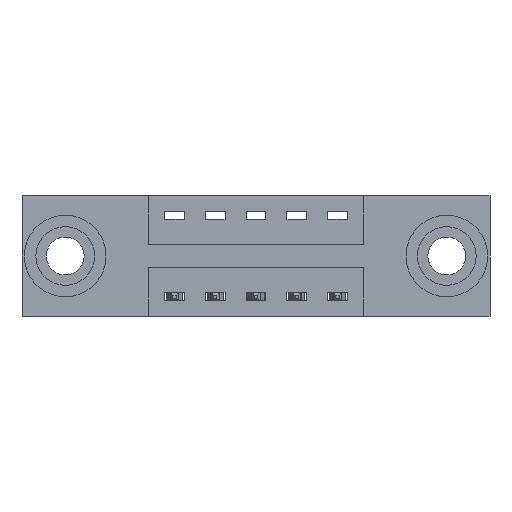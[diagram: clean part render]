
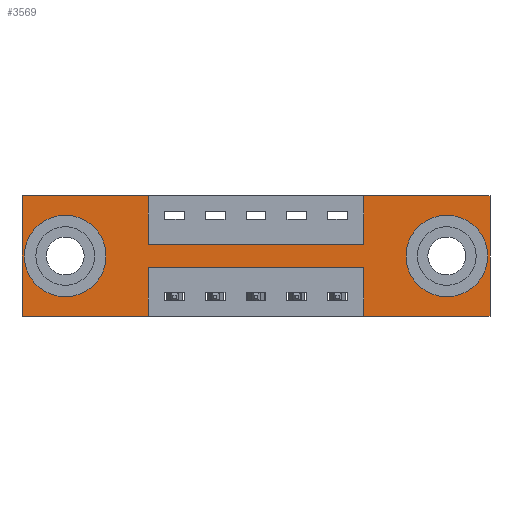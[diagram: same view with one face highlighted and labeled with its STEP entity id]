
A CAD part, front view. The second image highlights one B-rep face of the part: STEP entity #3569.
In plain terms, the highlighted planar face has unit normal (0, -1, 0).
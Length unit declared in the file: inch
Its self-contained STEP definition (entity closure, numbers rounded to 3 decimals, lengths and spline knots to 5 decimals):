
#14 = DIRECTION ( 'NONE',  ( 0., 1., 0. ) ) ;
#58 = VECTOR ( 'NONE', #2549, 39.37008 ) ;
#87 = DIRECTION ( 'NONE',  ( 0., 1., 0. ) ) ;
#312 = VERTEX_POINT ( 'NONE', #4707 ) ;
#434 = DIRECTION ( 'NONE',  ( 1., 0., 0. ) ) ;
#550 = DIRECTION ( 'NONE',  ( 0., 0., -1. ) ) ;
#617 = CARTESIAN_POINT ( 'NONE',  ( 0., 0., -0.37 ) ) ;
#631 = CIRCLE ( 'NONE', #5058, 0.078 ) ;
#636 = VECTOR ( 'NONE', #8516, 39.37008 ) ;
#1135 = VERTEX_POINT ( 'NONE', #1480 ) ;
#1148 = VERTEX_POINT ( 'NONE', #3266 ) ;
#1238 = VERTEX_POINT ( 'NONE', #4792 ) ;
#1344 = VECTOR ( 'NONE', #3670, 39.37008 ) ;
#1382 = CARTESIAN_POINT ( 'NONE',  ( 0., 0., -0.37 ) ) ;
#1480 = CARTESIAN_POINT ( 'NONE',  ( 1.0475, 0., 0. ) ) ;
#1633 = CIRCLE ( 'NONE', #2743, 0.078 ) ;
#1682 = LINE ( 'NONE', #617, #3852 ) ;
#1690 = EDGE_CURVE ( 'NONE', #5022, #4875, #1633, .T. ) ;
#1745 = VECTOR ( 'NONE', #2656, 39.37008 ) ;
#1761 = EDGE_CURVE ( 'NONE', #1135, #3083, #7922, .T. ) ;
#1864 = CARTESIAN_POINT ( 'NONE',  ( 0.3875, 0., -0.37 ) ) ;
#1916 = EDGE_LOOP ( 'NONE', ( #6002, #4593, #3584, #3527, #2947, #2757, #2307, #5243, #5201, #5235, #5082, #5350 ) ) ;
#1921 = CARTESIAN_POINT ( 'NONE',  ( 1.0475, 0., -0.37 ) ) ;
#1949 = CARTESIAN_POINT ( 'NONE',  ( 0., 0., -0.37 ) ) ;
#2166 = VECTOR ( 'NONE', #3898, 39.37008 ) ;
#2168 = CARTESIAN_POINT ( 'NONE',  ( 1.435, 0., 0. ) ) ;
#2193 = CARTESIAN_POINT ( 'NONE',  ( 0.3875, 0., -0.15 ) ) ;
#2196 = PLANE ( 'NONE',  #7880 ) ;
#2232 = CIRCLE ( 'NONE', #8319, 0.078 ) ;
#2291 = LINE ( 'NONE', #4595, #8593 ) ;
#2293 = EDGE_CURVE ( 'NONE', #8522, #1135, #6394, .T. ) ;
#2307 = ORIENTED_EDGE ( 'NONE', *, *, #2293, .F. ) ;
#2315 = FACE_BOUND ( 'NONE', #4770, .T. ) ;
#2337 = LINE ( 'NONE', #2193, #8637 ) ;
#2549 = DIRECTION ( 'NONE',  ( 0., 0., -1. ) ) ;
#2567 = LINE ( 'NONE', #3282, #58 ) ;
#2619 = CARTESIAN_POINT ( 'NONE',  ( 0.3875, 0., -0.22 ) ) ;
#2639 = CARTESIAN_POINT ( 'NONE',  ( 0.1325, 0., -0.263 ) ) ;
#2656 = DIRECTION ( 'NONE',  ( 0., 0., 1. ) ) ;
#2743 = AXIS2_PLACEMENT_3D ( 'NONE', #6141, #3408, #3191 ) ;
#2757 = ORIENTED_EDGE ( 'NONE', *, *, #1761, .F. ) ;
#2947 = ORIENTED_EDGE ( 'NONE', *, *, #8371, .F. ) ;
#3083 = VERTEX_POINT ( 'NONE', #2168 ) ;
#3154 = CARTESIAN_POINT ( 'NONE',  ( 0.3875, 0., 0. ) ) ;
#3191 = DIRECTION ( 'NONE',  ( 0., 0., 1. ) ) ;
#3193 = DIRECTION ( 'NONE',  ( 0., 0., -1. ) ) ;
#3266 = CARTESIAN_POINT ( 'NONE',  ( 1.3025, 0., -0.107 ) ) ;
#3282 = CARTESIAN_POINT ( 'NONE',  ( 0.3875, 0., -0.37 ) ) ;
#3408 = DIRECTION ( 'NONE',  ( 0., 1., 0. ) ) ;
#3461 = CARTESIAN_POINT ( 'NONE',  ( 1.0475, 0., 0. ) ) ;
#3478 = CARTESIAN_POINT ( 'NONE',  ( 0., 0., 0. ) ) ;
#3527 = ORIENTED_EDGE ( 'NONE', *, *, #4435, .F. ) ;
#3569 = ADVANCED_FACE ( 'NONE', ( #2315, #7407, #3978 ), #2196, .T. ) ;
#3582 = CARTESIAN_POINT ( 'NONE',  ( 0.3875, 0., -0.22 ) ) ;
#3584 = ORIENTED_EDGE ( 'NONE', *, *, #8078, .F. ) ;
#3670 = DIRECTION ( 'NONE',  ( 0., 0., -1. ) ) ;
#3748 = CIRCLE ( 'NONE', #7837, 0.078 ) ;
#3852 = VECTOR ( 'NONE', #5043, 39.37008 ) ;
#3898 = DIRECTION ( 'NONE',  ( 0., 0., 1. ) ) ;
#3944 = LINE ( 'NONE', #4159, #7181 ) ;
#3958 = EDGE_CURVE ( 'NONE', #7467, #1148, #3748, .T. ) ;
#3978 = FACE_OUTER_BOUND ( 'NONE', #1916, .T. ) ;
#4049 = DIRECTION ( 'NONE',  ( -1., 0., 0. ) ) ;
#4092 = ORIENTED_EDGE ( 'NONE', *, *, #3958, .T. ) ;
#4159 = CARTESIAN_POINT ( 'NONE',  ( 0., 0., 0. ) ) ;
#4255 = EDGE_LOOP ( 'NONE', ( #5183, #4677 ) ) ;
#4404 = LINE ( 'NONE', #1949, #7567 ) ;
#4421 = ORIENTED_EDGE ( 'NONE', *, *, #6792, .T. ) ;
#4435 = EDGE_CURVE ( 'NONE', #4826, #312, #1682, .T. ) ;
#4475 = CARTESIAN_POINT ( 'NONE',  ( 1.3025, 0., -0.185 ) ) ;
#4543 = CARTESIAN_POINT ( 'NONE',  ( 0.1325, 0., -0.185 ) ) ;
#4593 = ORIENTED_EDGE ( 'NONE', *, *, #8765, .F. ) ;
#4595 = CARTESIAN_POINT ( 'NONE',  ( 0.3875, 0., 0. ) ) ;
#4640 = EDGE_CURVE ( 'NONE', #5404, #5524, #2291, .T. ) ;
#4677 = ORIENTED_EDGE ( 'NONE', *, *, #8504, .T. ) ;
#4707 = CARTESIAN_POINT ( 'NONE',  ( 1.0475, 0., -0.37 ) ) ;
#4770 = EDGE_LOOP ( 'NONE', ( #4421, #4092 ) ) ;
#4792 = CARTESIAN_POINT ( 'NONE',  ( 1.0475, 0., -0.22 ) ) ;
#4826 = VERTEX_POINT ( 'NONE', #7833 ) ;
#4875 = VERTEX_POINT ( 'NONE', #2639 ) ;
#4951 = DIRECTION ( 'NONE',  ( 0., 1., 0. ) ) ;
#4991 = DIRECTION ( 'NONE',  ( 1., 0., 0. ) ) ;
#5022 = VERTEX_POINT ( 'NONE', #6173 ) ;
#5033 = CARTESIAN_POINT ( 'NONE',  ( 1.3025, 0., -0.263 ) ) ;
#5043 = DIRECTION ( 'NONE',  ( -1., 0., 0. ) ) ;
#5058 = AXIS2_PLACEMENT_3D ( 'NONE', #4475, #14, #5138 ) ;
#5082 = ORIENTED_EDGE ( 'NONE', *, *, #6207, .F. ) ;
#5138 = DIRECTION ( 'NONE',  ( 0., 0., -1. ) ) ;
#5183 = ORIENTED_EDGE ( 'NONE', *, *, #1690, .T. ) ;
#5195 = DIRECTION ( 'NONE',  ( 0., 0., 1. ) ) ;
#5201 = ORIENTED_EDGE ( 'NONE', *, *, #4640, .F. ) ;
#5235 = ORIENTED_EDGE ( 'NONE', *, *, #5640, .F. ) ;
#5243 = ORIENTED_EDGE ( 'NONE', *, *, #8278, .F. ) ;
#5279 = CARTESIAN_POINT ( 'NONE',  ( 0., 0., 0. ) ) ;
#5350 = ORIENTED_EDGE ( 'NONE', *, *, #5616, .F. ) ;
#5404 = VERTEX_POINT ( 'NONE', #3154 ) ;
#5524 = VERTEX_POINT ( 'NONE', #7776 ) ;
#5616 = EDGE_CURVE ( 'NONE', #7134, #7195, #4404, .T. ) ;
#5640 = EDGE_CURVE ( 'NONE', #7286, #5404, #3944, .T. ) ;
#6002 = ORIENTED_EDGE ( 'NONE', *, *, #7062, .F. ) ;
#6141 = CARTESIAN_POINT ( 'NONE',  ( 0.1325, 0., -0.185 ) ) ;
#6173 = CARTESIAN_POINT ( 'NONE',  ( 0.1325, 0., -0.107 ) ) ;
#6207 = EDGE_CURVE ( 'NONE', #7195, #7286, #7562, .T. ) ;
#6394 = LINE ( 'NONE', #3461, #7629 ) ;
#6466 = CARTESIAN_POINT ( 'NONE',  ( 1.0475, 0., -0.15 ) ) ;
#6673 = LINE ( 'NONE', #6941, #1344 ) ;
#6784 = DIRECTION ( 'NONE',  ( 0., 0., 1. ) ) ;
#6792 = EDGE_CURVE ( 'NONE', #1148, #7467, #631, .T. ) ;
#6893 = DIRECTION ( 'NONE',  ( 0., 0., -1. ) ) ;
#6941 = CARTESIAN_POINT ( 'NONE',  ( 1.435, 0., 0. ) ) ;
#7062 = EDGE_CURVE ( 'NONE', #8293, #7134, #2567, .T. ) ;
#7134 = VERTEX_POINT ( 'NONE', #1864 ) ;
#7148 = LINE ( 'NONE', #1921, #1745 ) ;
#7181 = VECTOR ( 'NONE', #434, 39.37008 ) ;
#7195 = VERTEX_POINT ( 'NONE', #7920 ) ;
#7229 = LINE ( 'NONE', #2619, #8628 ) ;
#7286 = VERTEX_POINT ( 'NONE', #3478 ) ;
#7322 = DIRECTION ( 'NONE',  ( -1., 0., 0. ) ) ;
#7407 = FACE_BOUND ( 'NONE', #4255, .T. ) ;
#7467 = VERTEX_POINT ( 'NONE', #5033 ) ;
#7562 = LINE ( 'NONE', #5279, #2166 ) ;
#7567 = VECTOR ( 'NONE', #7322, 39.37008 ) ;
#7629 = VECTOR ( 'NONE', #6784, 39.37008 ) ;
#7776 = CARTESIAN_POINT ( 'NONE',  ( 0.3875, 0., -0.15 ) ) ;
#7833 = CARTESIAN_POINT ( 'NONE',  ( 1.435, 0., -0.37 ) ) ;
#7837 = AXIS2_PLACEMENT_3D ( 'NONE', #8638, #4951, #550 ) ;
#7880 = AXIS2_PLACEMENT_3D ( 'NONE', #1382, #8674, #6893 ) ;
#7920 = CARTESIAN_POINT ( 'NONE',  ( 0., 0., -0.37 ) ) ;
#7922 = LINE ( 'NONE', #8497, #636 ) ;
#8078 = EDGE_CURVE ( 'NONE', #312, #1238, #7148, .T. ) ;
#8278 = EDGE_CURVE ( 'NONE', #5524, #8522, #2337, .T. ) ;
#8293 = VERTEX_POINT ( 'NONE', #3582 ) ;
#8319 = AXIS2_PLACEMENT_3D ( 'NONE', #4543, #87, #5195 ) ;
#8371 = EDGE_CURVE ( 'NONE', #3083, #4826, #6673, .T. ) ;
#8497 = CARTESIAN_POINT ( 'NONE',  ( 0., 0., 0. ) ) ;
#8504 = EDGE_CURVE ( 'NONE', #4875, #5022, #2232, .T. ) ;
#8516 = DIRECTION ( 'NONE',  ( 1., 0., 0. ) ) ;
#8522 = VERTEX_POINT ( 'NONE', #6466 ) ;
#8593 = VECTOR ( 'NONE', #3193, 39.37008 ) ;
#8628 = VECTOR ( 'NONE', #4049, 39.37008 ) ;
#8637 = VECTOR ( 'NONE', #4991, 39.37008 ) ;
#8638 = CARTESIAN_POINT ( 'NONE',  ( 1.3025, 0., -0.185 ) ) ;
#8674 = DIRECTION ( 'NONE',  ( 0., -1., 0. ) ) ;
#8765 = EDGE_CURVE ( 'NONE', #1238, #8293, #7229, .T. ) ;
